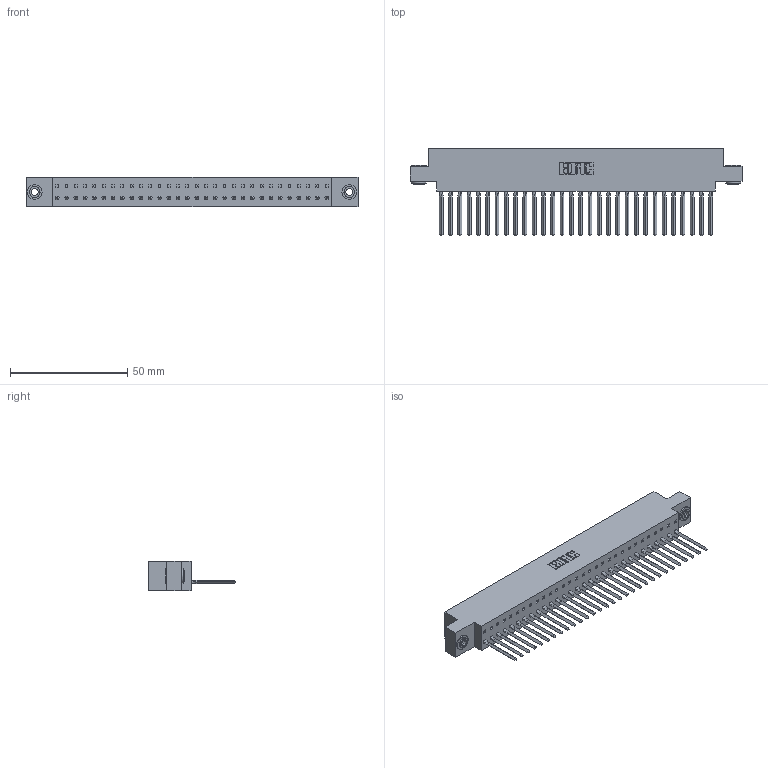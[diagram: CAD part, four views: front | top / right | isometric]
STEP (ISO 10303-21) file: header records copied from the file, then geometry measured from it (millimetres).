
FILE_DESCRIPTION (( 'STEP AP203' ), '1' );
FILE_NAME ('317-030-541-603.STEP', '2020-02-27T20:13:11', ( '' ), ( '' ), 'SwSTEP 2.0', 'SolidWorks 2016', '' );
FILE_SCHEMA (( 'CONFIG_CONTROL_DESIGN' ));
Length unit declared in the file: inch
Products named in the file (4): 345-250-002_345-250-002-102; 317 Part_.156 Dia - TH; 317-290-002_541; 317-030-541-603
Assembly tree (33 placements, depth 2):
  317-030-541-603
    317 Part_.156 Dia - TH
    317-290-002_541  x30
    345-250-002_345-250-002-102  x2
Bounding box: 141.58 x 37.34 x 12.7 mm (x, y, z)
Volume: 22609.9 mm3; surface area: 31763.9 mm2
Topology: 33 solids, 33 shells, 4700 faces, 13371 edges, 8690 vertices
Faces by surface type: plane 3788, cylinder 784, bspline 120, cone 8
Entity records: 46277 total; most frequent: CARTESIAN_POINT 8830, ORIENTED_EDGE 8106, DIRECTION 6691, EDGE_CURVE 4053, VECTOR 3665, LINE 3665, VERTEX_POINT 2692, AXIS2_PLACEMENT_3D 1513
